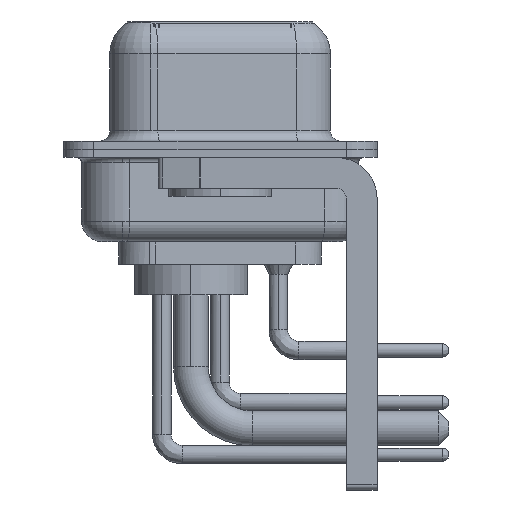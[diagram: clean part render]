
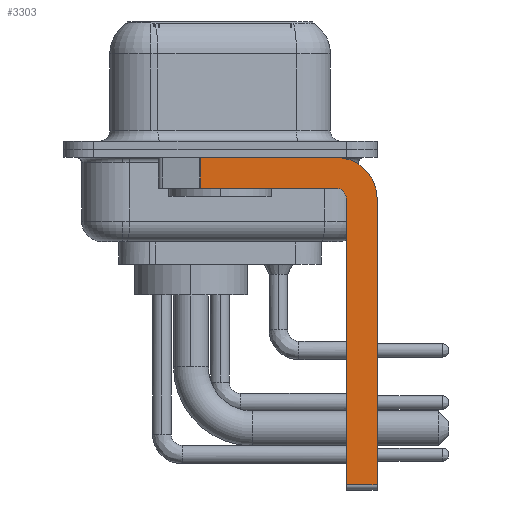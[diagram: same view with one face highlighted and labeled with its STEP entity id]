
A CAD part, left-side view. The second image highlights one B-rep face of the part: STEP entity #3303.
In plain terms, the highlighted planar face has unit normal (-1, 0, 0).
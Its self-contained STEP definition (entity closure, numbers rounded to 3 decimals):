
#529 = LINE ( 'NONE', #19075, #27077 ) ;
#555 = CARTESIAN_POINT ( 'NONE',  ( -2.9, -7.65, -2.4 ) ) ;
#2168 = VERTEX_POINT ( 'NONE', #555 ) ;
#3303 = ADVANCED_FACE ( 'NONE', ( #26835 ), #3807, .F. ) ;
#3595 = CIRCLE ( 'NONE', #28905, 0.5 ) ;
#3807 = PLANE ( 'NONE',  #16165 ) ;
#3823 = CARTESIAN_POINT ( 'NONE',  ( -2.9, 3., -0.4 ) ) ;
#3952 = CARTESIAN_POINT ( 'NONE',  ( -2.9, -5.65, -1.9 ) ) ;
#4487 = EDGE_CURVE ( 'NONE', #12995, #12048, #19962, .T. ) ;
#4716 = EDGE_LOOP ( 'NONE', ( #15726, #8986, #29694, #27577, #26171, #18381, #15081, #25466 ) ) ;
#4760 = VECTOR ( 'NONE', #19954, 1000. ) ;
#5469 = EDGE_CURVE ( 'NONE', #19790, #14602, #3595, .T. ) ;
#5925 = VECTOR ( 'NONE', #23954, 1000. ) ;
#7534 = CARTESIAN_POINT ( 'NONE',  ( -2.9, -5.65, -2.4 ) ) ;
#8274 = LINE ( 'NONE', #23967, #27233 ) ;
#8986 = ORIENTED_EDGE ( 'NONE', *, *, #24987, .T. ) ;
#9593 = EDGE_CURVE ( 'NONE', #2168, #24502, #11189, .T. ) ;
#10193 = CARTESIAN_POINT ( 'NONE',  ( -2.9, -7.65, -16.35 ) ) ;
#11189 = LINE ( 'NONE', #13611, #27934 ) ;
#11844 = CARTESIAN_POINT ( 'NONE',  ( -2.9, -6.15, -16.35 ) ) ;
#12048 = VERTEX_POINT ( 'NONE', #24991 ) ;
#12733 = EDGE_CURVE ( 'NONE', #28104, #24502, #529, .T. ) ;
#12894 = DIRECTION ( 'NONE',  ( 0., 0., 1. ) ) ;
#12995 = VERTEX_POINT ( 'NONE', #15719 ) ;
#13611 = CARTESIAN_POINT ( 'NONE',  ( -2.9, -7.65, -2.4 ) ) ;
#14569 = EDGE_CURVE ( 'NONE', #14602, #19787, #26999, .T. ) ;
#14602 = VERTEX_POINT ( 'NONE', #22245 ) ;
#15081 = ORIENTED_EDGE ( 'NONE', *, *, #9593, .F. ) ;
#15182 = DIRECTION ( 'NONE',  ( -1., 0., 0. ) ) ;
#15242 = CARTESIAN_POINT ( 'NONE',  ( -2.9, -5.65, -2.4 ) ) ;
#15537 = DIRECTION ( 'NONE',  ( 0., 0., -1. ) ) ;
#15719 = CARTESIAN_POINT ( 'NONE',  ( -2.9, 0.978, -0.4 ) ) ;
#15726 = ORIENTED_EDGE ( 'NONE', *, *, #4487, .F. ) ;
#16165 = AXIS2_PLACEMENT_3D ( 'NONE', #15242, #20092, #15537 ) ;
#16818 = DIRECTION ( 'NONE',  ( 1., 0., 0. ) ) ;
#17402 = EDGE_CURVE ( 'NONE', #28104, #19790, #28552, .T. ) ;
#17585 = CIRCLE ( 'NONE', #18539, 2. ) ;
#18381 = ORIENTED_EDGE ( 'NONE', *, *, #12733, .T. ) ;
#18539 = AXIS2_PLACEMENT_3D ( 'NONE', #7534, #16818, #21982 ) ;
#19072 = CARTESIAN_POINT ( 'NONE',  ( -2.9, -6.15, -16.6 ) ) ;
#19075 = CARTESIAN_POINT ( 'NONE',  ( -2.9, -5.65, -16.35 ) ) ;
#19787 = VERTEX_POINT ( 'NONE', #26807 ) ;
#19790 = VERTEX_POINT ( 'NONE', #24813 ) ;
#19954 = DIRECTION ( 'NONE',  ( 0., 1., 0. ) ) ;
#19962 = LINE ( 'NONE', #3823, #20228 ) ;
#20092 = DIRECTION ( 'NONE',  ( 1., 0., 0. ) ) ;
#20228 = VECTOR ( 'NONE', #26710, 1000. ) ;
#21669 = DIRECTION ( 'NONE',  ( 0., 0., -1. ) ) ;
#21982 = DIRECTION ( 'NONE',  ( 0., 0., -1. ) ) ;
#22245 = CARTESIAN_POINT ( 'NONE',  ( -2.9, -5.65, -1.9 ) ) ;
#22606 = DIRECTION ( 'NONE',  ( 0., 0., -1. ) ) ;
#23954 = DIRECTION ( 'NONE',  ( 0., 0., 1. ) ) ;
#23967 = CARTESIAN_POINT ( 'NONE',  ( -2.9, 0.978, -1.9 ) ) ;
#24484 = CARTESIAN_POINT ( 'NONE',  ( -2.9, -5.65, -2.4 ) ) ;
#24502 = VERTEX_POINT ( 'NONE', #10193 ) ;
#24813 = CARTESIAN_POINT ( 'NONE',  ( -2.9, -6.15, -2.4 ) ) ;
#24987 = EDGE_CURVE ( 'NONE', #12995, #19787, #8274, .T. ) ;
#24991 = CARTESIAN_POINT ( 'NONE',  ( -2.9, -5.65, -0.4 ) ) ;
#25466 = ORIENTED_EDGE ( 'NONE', *, *, #27277, .F. ) ;
#26171 = ORIENTED_EDGE ( 'NONE', *, *, #17402, .F. ) ;
#26710 = DIRECTION ( 'NONE',  ( 0., -1., 0. ) ) ;
#26807 = CARTESIAN_POINT ( 'NONE',  ( -2.9, 0.978, -1.9 ) ) ;
#26835 = FACE_OUTER_BOUND ( 'NONE', #4716, .T. ) ;
#26999 = LINE ( 'NONE', #3952, #4760 ) ;
#27077 = VECTOR ( 'NONE', #28406, 1000. ) ;
#27233 = VECTOR ( 'NONE', #21669, 1000. ) ;
#27277 = EDGE_CURVE ( 'NONE', #12048, #2168, #17585, .T. ) ;
#27577 = ORIENTED_EDGE ( 'NONE', *, *, #5469, .F. ) ;
#27934 = VECTOR ( 'NONE', #22606, 1000. ) ;
#28104 = VERTEX_POINT ( 'NONE', #11844 ) ;
#28406 = DIRECTION ( 'NONE',  ( 0., -1., 0. ) ) ;
#28552 = LINE ( 'NONE', #19072, #5925 ) ;
#28905 = AXIS2_PLACEMENT_3D ( 'NONE', #24484, #15182, #12894 ) ;
#29694 = ORIENTED_EDGE ( 'NONE', *, *, #14569, .F. ) ;
